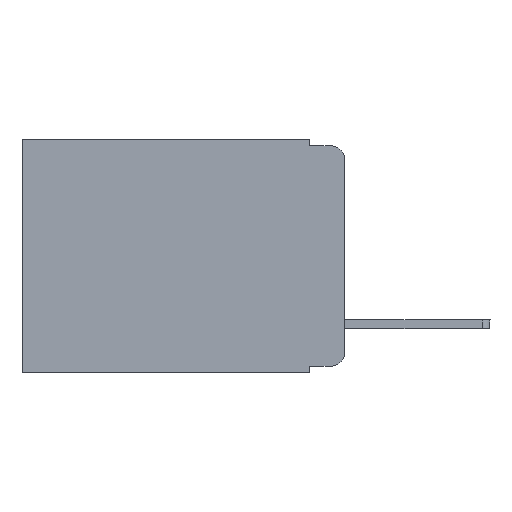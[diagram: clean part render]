
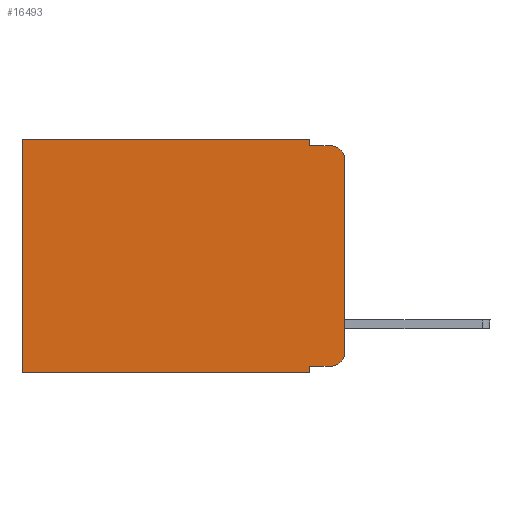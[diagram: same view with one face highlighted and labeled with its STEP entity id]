
A CAD part, left-side view. The second image highlights one B-rep face of the part: STEP entity #16493.
In plain terms, the highlighted planar face has unit normal (-1, 0, 0).
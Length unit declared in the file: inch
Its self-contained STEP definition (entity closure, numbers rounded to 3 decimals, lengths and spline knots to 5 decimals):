
#403 = ORIENTED_EDGE ( 'NONE', *, *, #16498, .F. ) ;
#489 = EDGE_LOOP ( 'NONE', ( #403, #11100, #1326, #6432, #14433, #10468, #8091, #10425, #16071, #16559 ) ) ;
#508 = EDGE_CURVE ( 'NONE', #15517, #12906, #5187, .T. ) ;
#764 = DIRECTION ( 'NONE',  ( -1., 0., 0. ) ) ;
#1197 = CARTESIAN_POINT ( 'NONE',  ( 0.298, 0.473, 0. ) ) ;
#1242 = VECTOR ( 'NONE', #6018, 39.37008 ) ;
#1271 = DIRECTION ( 'NONE',  ( 0., 1., 0. ) ) ;
#1326 = ORIENTED_EDGE ( 'NONE', *, *, #12327, .F. ) ;
#1821 = CARTESIAN_POINT ( 'NONE',  ( 0.298, 0.02, -0.01 ) ) ;
#2242 = EDGE_CURVE ( 'NONE', #16459, #12951, #4359, .T. ) ;
#2276 = DIRECTION ( 'NONE',  ( 0., 0., -1. ) ) ;
#2798 = VECTOR ( 'NONE', #14750, 39.37008 ) ;
#2885 = AXIS2_PLACEMENT_3D ( 'NONE', #13546, #764, #9863 ) ;
#2895 = CARTESIAN_POINT ( 'NONE',  ( 0.298, 0., -0.03 ) ) ;
#3366 = LINE ( 'NONE', #15084, #6009 ) ;
#4045 = DIRECTION ( 'NONE',  ( 0., 0., -1. ) ) ;
#4359 = CIRCLE ( 'NONE', #14720, 0.02 ) ;
#4418 = CARTESIAN_POINT ( 'NONE',  ( 0.298, 0.051, 0. ) ) ;
#4443 = VECTOR ( 'NONE', #15245, 39.37008 ) ;
#4974 = EDGE_CURVE ( 'NONE', #9838, #8790, #11609, .T. ) ;
#5075 = CARTESIAN_POINT ( 'NONE',  ( 0.298, 0., -0.313 ) ) ;
#5187 = LINE ( 'NONE', #9261, #5582 ) ;
#5582 = VECTOR ( 'NONE', #4045, 39.37008 ) ;
#5813 = LINE ( 'NONE', #4418, #2798 ) ;
#5841 = VERTEX_POINT ( 'NONE', #12066 ) ;
#5865 = DIRECTION ( 'NONE',  ( 0., 0., -1. ) ) ;
#6009 = VECTOR ( 'NONE', #5865, 39.37008 ) ;
#6018 = DIRECTION ( 'NONE',  ( 0., -1., 0. ) ) ;
#6037 = PLANE ( 'NONE',  #6826 ) ;
#6432 = ORIENTED_EDGE ( 'NONE', *, *, #13179, .F. ) ;
#6826 = AXIS2_PLACEMENT_3D ( 'NONE', #9851, #7393, #2276 ) ;
#6915 = DIRECTION ( 'NONE',  ( 0., 0., -1. ) ) ;
#7393 = DIRECTION ( 'NONE',  ( 1., 0., 0. ) ) ;
#7601 = CARTESIAN_POINT ( 'NONE',  ( 0.298, 0., -0.343 ) ) ;
#7607 = CARTESIAN_POINT ( 'NONE',  ( 0.298, 0.051, -0.333 ) ) ;
#7615 = EDGE_CURVE ( 'NONE', #13555, #16459, #9862, .T. ) ;
#8091 = ORIENTED_EDGE ( 'NONE', *, *, #11134, .F. ) ;
#8141 = LINE ( 'NONE', #9570, #11175 ) ;
#8790 = VERTEX_POINT ( 'NONE', #1821 ) ;
#9261 = CARTESIAN_POINT ( 'NONE',  ( 0.298, 0.473, 0. ) ) ;
#9570 = CARTESIAN_POINT ( 'NONE',  ( 0.298, 0.051, 0. ) ) ;
#9592 = VERTEX_POINT ( 'NONE', #9994 ) ;
#9838 = VERTEX_POINT ( 'NONE', #2895 ) ;
#9851 = CARTESIAN_POINT ( 'NONE',  ( 0.298, 0., 0. ) ) ;
#9862 = LINE ( 'NONE', #11192, #11874 ) ;
#9863 = DIRECTION ( 'NONE',  ( 0., 0., -1. ) ) ;
#9994 = CARTESIAN_POINT ( 'NONE',  ( 0.298, 0.051, -0.01 ) ) ;
#10241 = CARTESIAN_POINT ( 'NONE',  ( 0.298, 0., 0. ) ) ;
#10425 = ORIENTED_EDGE ( 'NONE', *, *, #10513, .F. ) ;
#10468 = ORIENTED_EDGE ( 'NONE', *, *, #508, .T. ) ;
#10513 = EDGE_CURVE ( 'NONE', #13555, #10825, #8141, .T. ) ;
#10825 = VERTEX_POINT ( 'NONE', #16407 ) ;
#11077 = DIRECTION ( 'NONE',  ( 0., -1., 0. ) ) ;
#11100 = ORIENTED_EDGE ( 'NONE', *, *, #4974, .T. ) ;
#11134 = EDGE_CURVE ( 'NONE', #10825, #12906, #14530, .T. ) ;
#11170 = CARTESIAN_POINT ( 'NONE',  ( 0.298, 0.02, -0.313 ) ) ;
#11175 = VECTOR ( 'NONE', #6915, 39.37008 ) ;
#11192 = CARTESIAN_POINT ( 'NONE',  ( 0.298, 0.051, -0.333 ) ) ;
#11609 = CIRCLE ( 'NONE', #2885, 0.02 ) ;
#11720 = LINE ( 'NONE', #12689, #1242 ) ;
#11874 = VECTOR ( 'NONE', #11077, 39.37008 ) ;
#12066 = CARTESIAN_POINT ( 'NONE',  ( 0.298, 0.051, 0. ) ) ;
#12327 = EDGE_CURVE ( 'NONE', #9592, #8790, #11720, .T. ) ;
#12689 = CARTESIAN_POINT ( 'NONE',  ( 0.298, 0.051, -0.01 ) ) ;
#12844 = CARTESIAN_POINT ( 'NONE',  ( 0.298, 0.473, -0.343 ) ) ;
#12887 = FACE_OUTER_BOUND ( 'NONE', #489, .T. ) ;
#12906 = VERTEX_POINT ( 'NONE', #12844 ) ;
#12951 = VERTEX_POINT ( 'NONE', #5075 ) ;
#13179 = EDGE_CURVE ( 'NONE', #5841, #9592, #5813, .T. ) ;
#13546 = CARTESIAN_POINT ( 'NONE',  ( 0.298, 0.02, -0.03 ) ) ;
#13555 = VERTEX_POINT ( 'NONE', #7607 ) ;
#13687 = EDGE_CURVE ( 'NONE', #5841, #15517, #15373, .T. ) ;
#13902 = DIRECTION ( 'NONE',  ( -1., 0., 0. ) ) ;
#14433 = ORIENTED_EDGE ( 'NONE', *, *, #13687, .T. ) ;
#14530 = LINE ( 'NONE', #7601, #4443 ) ;
#14720 = AXIS2_PLACEMENT_3D ( 'NONE', #11170, #13902, #16389 ) ;
#14750 = DIRECTION ( 'NONE',  ( 0., 0., -1. ) ) ;
#14964 = CARTESIAN_POINT ( 'NONE',  ( 0.298, 0.02, -0.333 ) ) ;
#15084 = CARTESIAN_POINT ( 'NONE',  ( 0.298, 0., 0. ) ) ;
#15245 = DIRECTION ( 'NONE',  ( 0., 1., 0. ) ) ;
#15373 = LINE ( 'NONE', #10241, #15562 ) ;
#15517 = VERTEX_POINT ( 'NONE', #1197 ) ;
#15562 = VECTOR ( 'NONE', #1271, 39.37008 ) ;
#16071 = ORIENTED_EDGE ( 'NONE', *, *, #7615, .T. ) ;
#16389 = DIRECTION ( 'NONE',  ( 0., 0., -1. ) ) ;
#16407 = CARTESIAN_POINT ( 'NONE',  ( 0.298, 0.051, -0.343 ) ) ;
#16459 = VERTEX_POINT ( 'NONE', #14964 ) ;
#16493 = ADVANCED_FACE ( 'NONE', ( #12887 ), #6037, .F. ) ;
#16498 = EDGE_CURVE ( 'NONE', #9838, #12951, #3366, .T. ) ;
#16559 = ORIENTED_EDGE ( 'NONE', *, *, #2242, .T. ) ;
